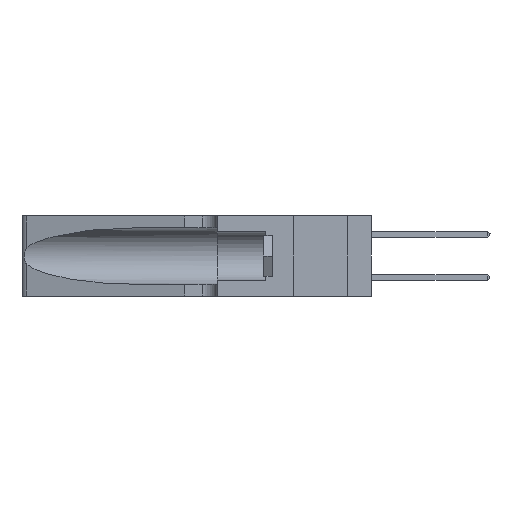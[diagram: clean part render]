
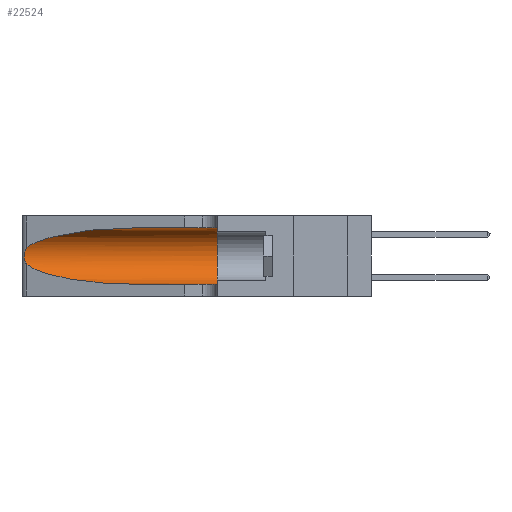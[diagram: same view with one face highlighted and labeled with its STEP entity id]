
A CAD part, left-side view. The second image highlights one B-rep face of the part: STEP entity #22524.
In plain terms, the highlighted cylindrical face has radius 3.308 mm (diameter 6.617 mm), a partial arc.
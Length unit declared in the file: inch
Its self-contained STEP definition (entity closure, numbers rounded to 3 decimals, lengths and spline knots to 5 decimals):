
#33 = B_SPLINE_CURVE_WITH_KNOTS ( 'NONE', 3,
 ( #12633, #10839, #10994, #12771, #14567, #16171, #7440, #7514, #3952, #1976, #2049, #17946, #19963, #14644 ),
 .UNSPECIFIED., .F., .F.,
 ( 4, 2, 2, 2, 2, 2, 4 ),
 ( 0., 0.00027, 0.00053, 0.00107, 0.0016, 0.00187, 0.00214 ),
 .UNSPECIFIED. ) ;
#330 = CARTESIAN_POINT ( 'NONE',  ( 0.1305, 0.35, 0.05475 ) ) ;
#365 = CARTESIAN_POINT ( 'NONE',  ( 0.1305, 0.72297, 0.05475 ) ) ;
#666 = CARTESIAN_POINT ( 'NONE',  ( 0.18966, 0.96281, 0.05475 ) ) ;
#718 = ORIENTED_EDGE ( 'NONE', *, *, #11160, .F. ) ;
#1051 = CYLINDRICAL_SURFACE ( 'NONE', #4692, 0.13025 ) ;
#1080 = ORIENTED_EDGE ( 'NONE', *, *, #14051, .T. ) ;
#1353 = VECTOR ( 'NONE', #12117, 39.37008 ) ;
#1976 = CARTESIAN_POINT ( 'NONE',  ( 0.25856, 1.23593, 0.16098 ) ) ;
#2049 = CARTESIAN_POINT ( 'NONE',  ( 0.25789, 1.23486, 0.15765 ) ) ;
#2332 = EDGE_CURVE ( 'NONE', #13825, #6196, #33, .T. ) ;
#2449 = FACE_OUTER_BOUND ( 'NONE', #17522, .T. ) ;
#3312 = CARTESIAN_POINT ( 'NONE',  ( 0.1305, 0.35, 0.31525 ) ) ;
#3532 = CARTESIAN_POINT ( 'NONE',  ( 0.1305, 0.72297, 0.05475 ) ) ;
#3952 = CARTESIAN_POINT ( 'NONE',  ( 0.26017, 1.23833, 0.17102 ) ) ;
#4617 = DIRECTION ( 'NONE',  ( 0., 0., -1. ) ) ;
#4692 = AXIS2_PLACEMENT_3D ( 'NONE', #19054, #13589, #4617 ) ;
#5236 = DIRECTION ( 'NONE',  ( 0., 0., 1. ) ) ;
#6196 = VERTEX_POINT ( 'NONE', #17935 ) ;
#6937 = CARTESIAN_POINT ( 'NONE',  ( 0.1305, 0.35, 0.185 ) ) ;
#6942 = CARTESIAN_POINT ( 'NONE',  ( 0.1305, 1.61858, 0.31525 ) ) ;
#7440 = CARTESIAN_POINT ( 'NONE',  ( 0.26075, 1.23896, 0.19203 ) ) ;
#7514 = CARTESIAN_POINT ( 'NONE',  ( 0.26075, 1.23896, 0.178 ) ) ;
#8586 = CARTESIAN_POINT ( 'NONE',  ( 0.1305, 0.72297, 0.31525 ) ) ;
#9362 = CARTESIAN_POINT ( 'NONE',  ( 0.25487, 1.22718, 0.22369 ) ) ;
#9384 = VERTEX_POINT ( 'NONE', #3312 ) ;
#10306 = VECTOR ( 'NONE', #22028, 39.37008 ) ;
#10839 = CARTESIAN_POINT ( 'NONE',  ( 0.25555, 1.22994, 0.2215 ) ) ;
#10994 = CARTESIAN_POINT ( 'NONE',  ( 0.25639, 1.23184, 0.21858 ) ) ;
#11160 = EDGE_CURVE ( 'NONE', #9384, #18227, #18954, .T. ) ;
#11240 = CARTESIAN_POINT ( 'NONE',  ( 0.2373, 1.15595, 0.08982 ) ) ;
#11313 = ORIENTED_EDGE ( 'NONE', *, *, #2332, .T. ) ;
#12059 =( BOUNDED_CURVE ( )  B_SPLINE_CURVE ( 3, ( #21877, #11240, #666, #365 ),
 .UNSPECIFIED., .F., .F. ) 
 B_SPLINE_CURVE_WITH_KNOTS ( ( 4, 4 ),
 ( 3.44316, 4.71239 ),
 .UNSPECIFIED. ) 
 CURVE ( )  GEOMETRIC_REPRESENTATION_ITEM ( )  RATIONAL_B_SPLINE_CURVE ( ( 1., 0.87, 0.87, 1. ) ) 
 REPRESENTATION_ITEM ( '' )  );
#12117 = DIRECTION ( 'NONE',  ( 0., -1., 0. ) ) ;
#12192 = VERTEX_POINT ( 'NONE', #3532 ) ;
#12258 = LINE ( 'NONE', #15050, #10306 ) ;
#12633 = CARTESIAN_POINT ( 'NONE',  ( 0.25487, 1.22718, 0.22369 ) ) ;
#12759 =( BOUNDED_CURVE ( )  B_SPLINE_CURVE ( 3, ( #13004, #13777, #19238, #17563 ),
 .UNSPECIFIED., .F., .F. ) 
 B_SPLINE_CURVE_WITH_KNOTS ( ( 4, 4 ),
 ( 1.5708, 2.84003 ),
 .UNSPECIFIED. ) 
 CURVE ( )  GEOMETRIC_REPRESENTATION_ITEM ( )  RATIONAL_B_SPLINE_CURVE ( ( 1., 0.87, 0.87, 1. ) ) 
 REPRESENTATION_ITEM ( '' )  );
#12771 = CARTESIAN_POINT ( 'NONE',  ( 0.25787, 1.23484, 0.2124 ) ) ;
#13004 = CARTESIAN_POINT ( 'NONE',  ( 0.1305, 0.72297, 0.31525 ) ) ;
#13589 = DIRECTION ( 'NONE',  ( 0., -1., 0. ) ) ;
#13614 = VERTEX_POINT ( 'NONE', #8586 ) ;
#13777 = CARTESIAN_POINT ( 'NONE',  ( 0.18966, 0.96281, 0.31525 ) ) ;
#13825 = VERTEX_POINT ( 'NONE', #9362 ) ;
#13909 = EDGE_CURVE ( 'NONE', #6196, #12192, #12059, .T. ) ;
#14051 = EDGE_CURVE ( 'NONE', #13614, #13825, #12759, .T. ) ;
#14567 = CARTESIAN_POINT ( 'NONE',  ( 0.25854, 1.2359, 0.20912 ) ) ;
#14644 = CARTESIAN_POINT ( 'NONE',  ( 0.25487, 1.22718, 0.14631 ) ) ;
#15050 = CARTESIAN_POINT ( 'NONE',  ( 0.1305, 1.61858, 0.05475 ) ) ;
#15319 = AXIS2_PLACEMENT_3D ( 'NONE', #6937, #22583, #5236 ) ;
#16171 = CARTESIAN_POINT ( 'NONE',  ( 0.26018, 1.23835, 0.19895 ) ) ;
#16655 = ORIENTED_EDGE ( 'NONE', *, *, #13909, .T. ) ;
#17104 = ORIENTED_EDGE ( 'NONE', *, *, #20745, .T. ) ;
#17522 = EDGE_LOOP ( 'NONE', ( #1080, #11313, #16655, #17104, #718, #22908 ) ) ;
#17563 = CARTESIAN_POINT ( 'NONE',  ( 0.25487, 1.22718, 0.22369 ) ) ;
#17935 = CARTESIAN_POINT ( 'NONE',  ( 0.25487, 1.22718, 0.14631 ) ) ;
#17946 = CARTESIAN_POINT ( 'NONE',  ( 0.25639, 1.23186, 0.15144 ) ) ;
#18116 = EDGE_CURVE ( 'NONE', #13614, #9384, #20220, .T. ) ;
#18227 = VERTEX_POINT ( 'NONE', #330 ) ;
#18954 = CIRCLE ( 'NONE', #15319, 0.13025 ) ;
#19054 = CARTESIAN_POINT ( 'NONE',  ( 0.1305, 1.61858, 0.185 ) ) ;
#19238 = CARTESIAN_POINT ( 'NONE',  ( 0.2373, 1.15595, 0.28018 ) ) ;
#19963 = CARTESIAN_POINT ( 'NONE',  ( 0.25555, 1.22993, 0.14849 ) ) ;
#20220 = LINE ( 'NONE', #6942, #1353 ) ;
#20745 = EDGE_CURVE ( 'NONE', #12192, #18227, #12258, .T. ) ;
#21877 = CARTESIAN_POINT ( 'NONE',  ( 0.25487, 1.22718, 0.14631 ) ) ;
#22028 = DIRECTION ( 'NONE',  ( 0., -1., 0. ) ) ;
#22524 = ADVANCED_FACE ( 'NONE', ( #2449 ), #1051, .F. ) ;
#22583 = DIRECTION ( 'NONE',  ( 0., 1., 0. ) ) ;
#22908 = ORIENTED_EDGE ( 'NONE', *, *, #18116, .F. ) ;
